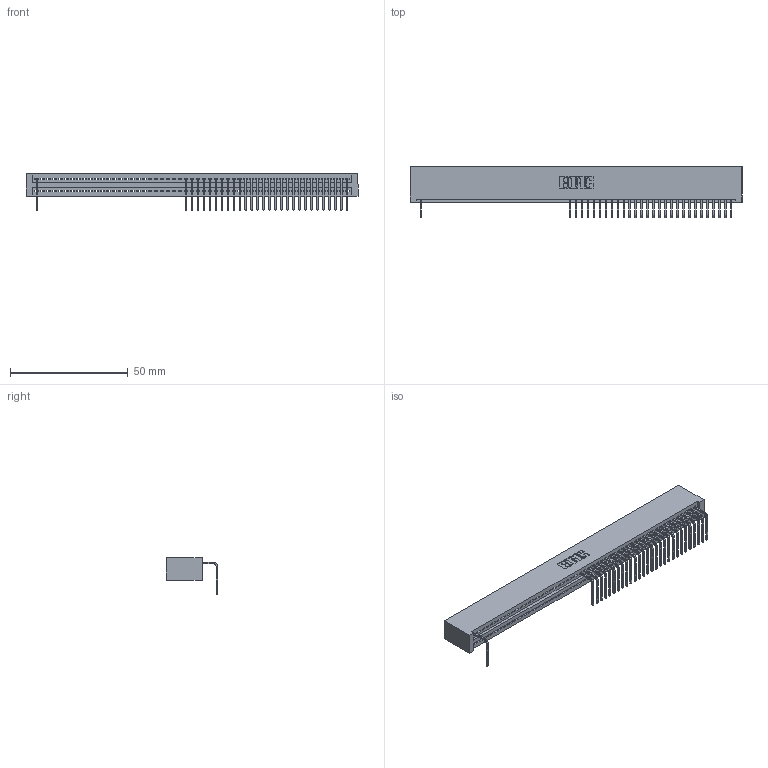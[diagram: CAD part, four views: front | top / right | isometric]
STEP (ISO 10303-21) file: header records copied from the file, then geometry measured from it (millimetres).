
FILE_DESCRIPTION (( 'STEP AP203' ), '1' );
FILE_NAME ('345-053-558-101.STEP', '2018-09-23T19:00:48', ( '' ), ( '' ), 'SwSTEP 2.0', 'SolidWorks 2016', '' );
FILE_SCHEMA (( 'CONFIG_CONTROL_DESIGN' ));
Length unit declared in the file: inch
Products named in the file (3): 345 Part_No Mounting Lugs; 345-292-001_558 Tail - 2; 345-053-558-101
Assembly tree (30 placements, depth 2):
  345-053-558-101
    345 Part_No Mounting Lugs
    345-292-001_558 Tail - 2  x29
Bounding box: 141.22 x 21.83 x 15.37 mm (x, y, z)
Volume: 13909.9 mm3; surface area: 17932.9 mm2
Topology: 30 solids, 30 shells, 2242 faces, 6891 edges, 4554 vertices
Faces by surface type: plane 1630, cylinder 612
Entity records: 37447 total; most frequent: ORIENTED_EDGE 6614, CARTESIAN_POINT 6603, DIRECTION 5717, EDGE_CURVE 3307, VECTOR 2971, LINE 2971, VERTEX_POINT 2202, AXIS2_PLACEMENT_3D 1373
